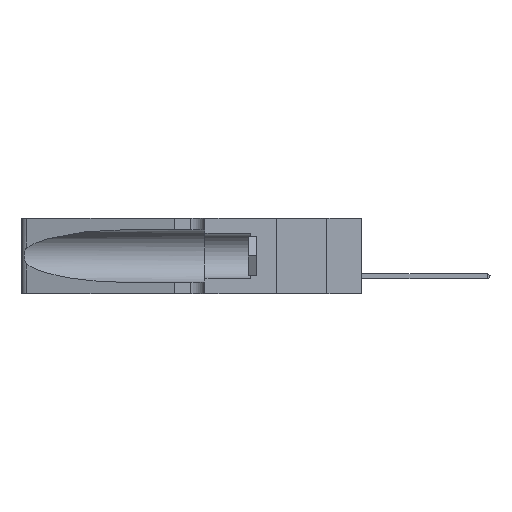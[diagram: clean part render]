
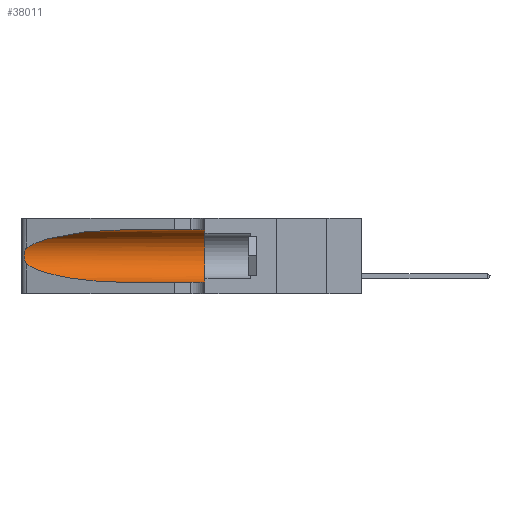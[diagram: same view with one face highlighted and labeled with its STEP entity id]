
A CAD part, left-side view. The second image highlights one B-rep face of the part: STEP entity #38011.
In plain terms, the highlighted cylindrical face has radius 3.308 mm (diameter 6.617 mm), a partial arc.
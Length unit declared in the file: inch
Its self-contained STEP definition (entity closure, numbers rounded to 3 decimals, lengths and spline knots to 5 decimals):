
#686 = B_SPLINE_CURVE_WITH_KNOTS ( 'NONE', 3,
 ( #49158, #18104, #25403, #48978, #33819, #49596, #37612, #17375, #36868, #2889, #6842, #5222, #21281, #36326 ),
 .UNSPECIFIED., .F., .F.,
 ( 4, 2, 2, 2, 2, 2, 4 ),
 ( 0., 0.00027, 0.00053, 0.00107, 0.0016, 0.00187, 0.00214 ),
 .UNSPECIFIED. ) ;
#1245 = DIRECTION ( 'NONE',  ( 0., 0., 1. ) ) ;
#2889 = CARTESIAN_POINT ( 'NONE',  ( 0.25856, 1.23593, 0.16098 ) ) ;
#3912 = ORIENTED_EDGE ( 'NONE', *, *, #47849, .T. ) ;
#3990 = VERTEX_POINT ( 'NONE', #22315 ) ;
#4005 =( BOUNDED_CURVE ( )  B_SPLINE_CURVE ( 3, ( #36637, #43758, #47848, #32347 ),
 .UNSPECIFIED., .F., .T. ) 
 B_SPLINE_CURVE_WITH_KNOTS ( ( 4, 4 ),
 ( 1.5708, 2.84003 ),
 .UNSPECIFIED. ) 
 CURVE ( )  GEOMETRIC_REPRESENTATION_ITEM ( )  RATIONAL_B_SPLINE_CURVE ( ( 1., 0.87, 0.87, 1. ) ) 
 REPRESENTATION_ITEM ( '' )  );
#4739 = ORIENTED_EDGE ( 'NONE', *, *, #35408, .F. ) ;
#5222 = CARTESIAN_POINT ( 'NONE',  ( 0.25639, 1.23186, 0.15144 ) ) ;
#6702 = CARTESIAN_POINT ( 'NONE',  ( 0.25487, 1.22718, 0.14631 ) ) ;
#6842 = CARTESIAN_POINT ( 'NONE',  ( 0.25789, 1.23486, 0.15765 ) ) ;
#7230 = CARTESIAN_POINT ( 'NONE',  ( 0.18966, 0.96281, 0.05475 ) ) ;
#7544 = CARTESIAN_POINT ( 'NONE',  ( 0.1305, 0.72297, 0.05475 ) ) ;
#8956 = VECTOR ( 'NONE', #23530, 39.37008 ) ;
#10783 = CARTESIAN_POINT ( 'NONE',  ( 0.25487, 1.22718, 0.22369 ) ) ;
#10999 = ORIENTED_EDGE ( 'NONE', *, *, #24854, .T. ) ;
#11060 = VECTOR ( 'NONE', #47051, 39.37008 ) ;
#14081 = CARTESIAN_POINT ( 'NONE',  ( 0.1305, 1.61858, 0.31525 ) ) ;
#16429 = VERTEX_POINT ( 'NONE', #44176 ) ;
#17375 = CARTESIAN_POINT ( 'NONE',  ( 0.26075, 1.23896, 0.178 ) ) ;
#17736 = EDGE_CURVE ( 'NONE', #18453, #32437, #686, .T. ) ;
#18104 = CARTESIAN_POINT ( 'NONE',  ( 0.25555, 1.22994, 0.2215 ) ) ;
#18453 = VERTEX_POINT ( 'NONE', #10783 ) ;
#18934 = FACE_OUTER_BOUND ( 'NONE', #33124, .T. ) ;
#21281 = CARTESIAN_POINT ( 'NONE',  ( 0.25555, 1.22993, 0.14849 ) ) ;
#21845 = CARTESIAN_POINT ( 'NONE',  ( 0.1305, 0.72297, 0.31525 ) ) ;
#22315 = CARTESIAN_POINT ( 'NONE',  ( 0.1305, 0.72297, 0.05475 ) ) ;
#23202 = CARTESIAN_POINT ( 'NONE',  ( 0.1305, 0.35, 0.05475 ) ) ;
#23530 = DIRECTION ( 'NONE',  ( 0., -1., 0. ) ) ;
#24661 = DIRECTION ( 'NONE',  ( 0., 1., 0. ) ) ;
#24854 = EDGE_CURVE ( 'NONE', #30241, #18453, #4005, .T. ) ;
#25403 = CARTESIAN_POINT ( 'NONE',  ( 0.25639, 1.23184, 0.21858 ) ) ;
#26736 = ORIENTED_EDGE ( 'NONE', *, *, #17736, .T. ) ;
#27637 = CARTESIAN_POINT ( 'NONE',  ( 0.1305, 1.61858, 0.05475 ) ) ;
#28222 = CARTESIAN_POINT ( 'NONE',  ( 0.1305, 1.61858, 0.185 ) ) ;
#29939 = ORIENTED_EDGE ( 'NONE', *, *, #37665, .F. ) ;
#29969 = CYLINDRICAL_SURFACE ( 'NONE', #43059, 0.13025 ) ;
#30241 = VERTEX_POINT ( 'NONE', #21845 ) ;
#30244 = EDGE_CURVE ( 'NONE', #32437, #3990, #36465, .T. ) ;
#32347 = CARTESIAN_POINT ( 'NONE',  ( 0.25487, 1.22718, 0.22369 ) ) ;
#32374 = CARTESIAN_POINT ( 'NONE',  ( 0.1305, 0.35, 0.185 ) ) ;
#32379 = CARTESIAN_POINT ( 'NONE',  ( 0.25487, 1.22718, 0.14631 ) ) ;
#32437 = VERTEX_POINT ( 'NONE', #32379 ) ;
#33124 = EDGE_LOOP ( 'NONE', ( #10999, #26736, #41235, #3912, #4739, #29939 ) ) ;
#33819 = CARTESIAN_POINT ( 'NONE',  ( 0.25854, 1.2359, 0.20912 ) ) ;
#35193 = AXIS2_PLACEMENT_3D ( 'NONE', #32374, #24661, #1245 ) ;
#35408 = EDGE_CURVE ( 'NONE', #16429, #46120, #49794, .T. ) ;
#35974 = LINE ( 'NONE', #14081, #11060 ) ;
#36236 = DIRECTION ( 'NONE',  ( 0., 0., -1. ) ) ;
#36326 = CARTESIAN_POINT ( 'NONE',  ( 0.25487, 1.22718, 0.14631 ) ) ;
#36465 =( BOUNDED_CURVE ( )  B_SPLINE_CURVE ( 3, ( #6702, #41854, #7230, #7544 ),
 .UNSPECIFIED., .F., .F. ) 
 B_SPLINE_CURVE_WITH_KNOTS ( ( 4, 4 ),
 ( 3.44316, 4.71239 ),
 .UNSPECIFIED. ) 
 CURVE ( )  GEOMETRIC_REPRESENTATION_ITEM ( )  RATIONAL_B_SPLINE_CURVE ( ( 1., 0.87, 0.87, 1. ) ) 
 REPRESENTATION_ITEM ( '' )  );
#36637 = CARTESIAN_POINT ( 'NONE',  ( 0.1305, 0.72297, 0.31525 ) ) ;
#36868 = CARTESIAN_POINT ( 'NONE',  ( 0.26017, 1.23833, 0.17102 ) ) ;
#37152 = LINE ( 'NONE', #27637, #8956 ) ;
#37612 = CARTESIAN_POINT ( 'NONE',  ( 0.26075, 1.23896, 0.19203 ) ) ;
#37665 = EDGE_CURVE ( 'NONE', #30241, #16429, #35974, .T. ) ;
#38011 = ADVANCED_FACE ( 'NONE', ( #18934 ), #29969, .F. ) ;
#41235 = ORIENTED_EDGE ( 'NONE', *, *, #30244, .T. ) ;
#41854 = CARTESIAN_POINT ( 'NONE',  ( 0.2373, 1.15595, 0.08982 ) ) ;
#43059 = AXIS2_PLACEMENT_3D ( 'NONE', #28222, #43864, #36236 ) ;
#43758 = CARTESIAN_POINT ( 'NONE',  ( 0.18966, 0.96281, 0.31525 ) ) ;
#43864 = DIRECTION ( 'NONE',  ( 0., -1., 0. ) ) ;
#44176 = CARTESIAN_POINT ( 'NONE',  ( 0.1305, 0.35, 0.31525 ) ) ;
#46120 = VERTEX_POINT ( 'NONE', #23202 ) ;
#47051 = DIRECTION ( 'NONE',  ( 0., -1., 0. ) ) ;
#47848 = CARTESIAN_POINT ( 'NONE',  ( 0.2373, 1.15595, 0.28018 ) ) ;
#47849 = EDGE_CURVE ( 'NONE', #3990, #46120, #37152, .T. ) ;
#48978 = CARTESIAN_POINT ( 'NONE',  ( 0.25787, 1.23484, 0.2124 ) ) ;
#49158 = CARTESIAN_POINT ( 'NONE',  ( 0.25487, 1.22718, 0.22369 ) ) ;
#49596 = CARTESIAN_POINT ( 'NONE',  ( 0.26018, 1.23835, 0.19895 ) ) ;
#49794 = CIRCLE ( 'NONE', #35193, 0.13025 ) ;
